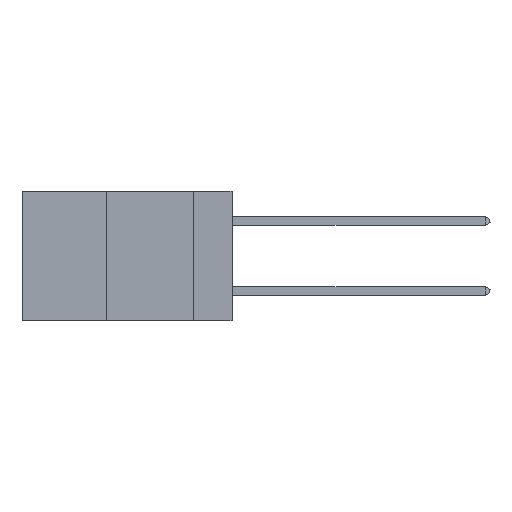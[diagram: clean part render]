
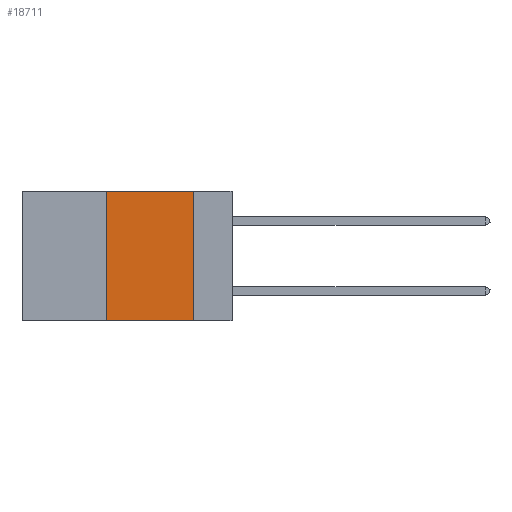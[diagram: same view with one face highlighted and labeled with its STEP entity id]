
A CAD part, left-side view. The second image highlights one B-rep face of the part: STEP entity #18711.
In plain terms, the highlighted planar face has unit normal (-1, 0, 0).
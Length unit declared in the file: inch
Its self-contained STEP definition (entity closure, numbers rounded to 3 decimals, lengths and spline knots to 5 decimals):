
#1389 = EDGE_CURVE ( 'NONE', #7914, #2313, #12963, .T. ) ;
#1953 = FACE_OUTER_BOUND ( 'NONE', #9311, .T. ) ;
#2204 = CARTESIAN_POINT ( 'NONE',  ( 0., 0.6, 0. ) ) ;
#2313 = VERTEX_POINT ( 'NONE', #21385 ) ;
#3080 = ORIENTED_EDGE ( 'NONE', *, *, #1389, .T. ) ;
#3311 = LINE ( 'NONE', #7478, #21029 ) ;
#3603 = CARTESIAN_POINT ( 'NONE',  ( 0., 0.6, 0. ) ) ;
#3709 = VECTOR ( 'NONE', #13594, 39.37008 ) ;
#3769 = LINE ( 'NONE', #3603, #7913 ) ;
#3979 = DIRECTION ( 'NONE',  ( 0., 0., -1. ) ) ;
#5171 = LINE ( 'NONE', #21293, #22278 ) ;
#6225 = ORIENTED_EDGE ( 'NONE', *, *, #21044, .F. ) ;
#7478 = CARTESIAN_POINT ( 'NONE',  ( 0., 0.11, 0. ) ) ;
#7913 = VECTOR ( 'NONE', #19094, 39.37008 ) ;
#7914 = VERTEX_POINT ( 'NONE', #10168 ) ;
#8170 = CARTESIAN_POINT ( 'NONE',  ( 0., 0.11, 0. ) ) ;
#8425 = CARTESIAN_POINT ( 'NONE',  ( 0., 0.6, -0.37 ) ) ;
#9311 = EDGE_LOOP ( 'NONE', ( #12847, #6225, #19904, #3080 ) ) ;
#10064 = VERTEX_POINT ( 'NONE', #16015 ) ;
#10168 = CARTESIAN_POINT ( 'NONE',  ( 0., 0.36, -0.37 ) ) ;
#10181 = EDGE_CURVE ( 'NONE', #7914, #10064, #5171, .T. ) ;
#10719 = AXIS2_PLACEMENT_3D ( 'NONE', #2204, #14377, #3979 ) ;
#10920 = DIRECTION ( 'NONE',  ( 0., 0., -1. ) ) ;
#12648 = PLANE ( 'NONE',  #10719 ) ;
#12847 = ORIENTED_EDGE ( 'NONE', *, *, #19298, .F. ) ;
#12963 = LINE ( 'NONE', #8425, #3709 ) ;
#13594 = DIRECTION ( 'NONE',  ( 0., -1., 0. ) ) ;
#14377 = DIRECTION ( 'NONE',  ( 1., 0., 0. ) ) ;
#14580 = DIRECTION ( 'NONE',  ( 0., 0., 1. ) ) ;
#15086 = VERTEX_POINT ( 'NONE', #8170 ) ;
#16015 = CARTESIAN_POINT ( 'NONE',  ( 0., 0.36, 0. ) ) ;
#18711 = ADVANCED_FACE ( 'NONE', ( #1953 ), #12648, .F. ) ;
#19094 = DIRECTION ( 'NONE',  ( 0., -1., 0. ) ) ;
#19298 = EDGE_CURVE ( 'NONE', #15086, #2313, #3311, .T. ) ;
#19904 = ORIENTED_EDGE ( 'NONE', *, *, #10181, .F. ) ;
#21029 = VECTOR ( 'NONE', #10920, 39.37008 ) ;
#21044 = EDGE_CURVE ( 'NONE', #10064, #15086, #3769, .T. ) ;
#21293 = CARTESIAN_POINT ( 'NONE',  ( 0., 0.36, 0. ) ) ;
#21385 = CARTESIAN_POINT ( 'NONE',  ( 0., 0.11, -0.37 ) ) ;
#22278 = VECTOR ( 'NONE', #14580, 39.37008 ) ;
